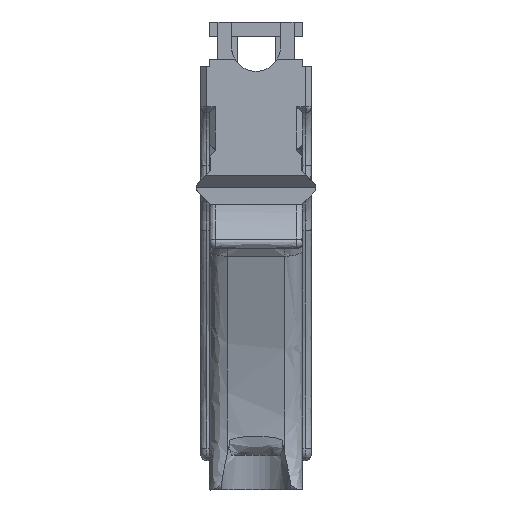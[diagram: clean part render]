
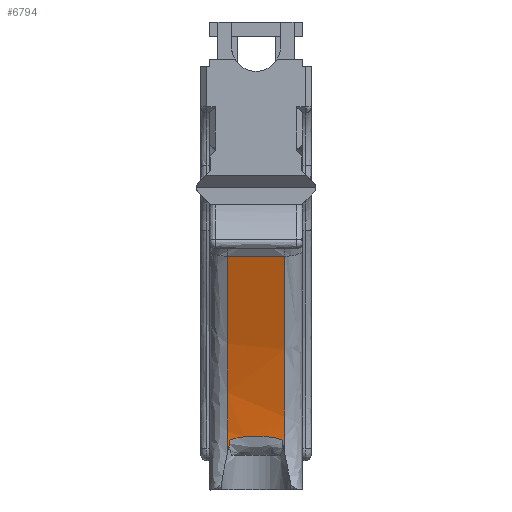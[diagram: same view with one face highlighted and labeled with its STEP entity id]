
A CAD part, front view. The second image highlights one B-rep face of the part: STEP entity #6794.
In plain terms, the highlighted free-form (B-spline) face has degree [5, 1] with [25, 2] control points.
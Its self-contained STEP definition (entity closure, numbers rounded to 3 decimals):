
#52=(
BOUNDED_SURFACE()
B_SPLINE_SURFACE(5,1,((#10452,#10453),(#10454,#10455),(#10456,#10457),(#10458,
#10459),(#10460,#10461),(#10462,#10463),(#10464,#10465),(#10466,#10467),
(#10468,#10469),(#10470,#10471),(#10472,#10473),(#10474,#10475),(#10476,
#10477),(#10478,#10479),(#10480,#10481),(#10482,#10483),(#10484,#10485),
(#10486,#10487),(#10488,#10489),(#10490,#10491),(#10492,#10493),(#10494,
#10495),(#10496,#10497),(#10498,#10499),(#10500,#10501)),.UNSPECIFIED.,
 .F.,.F.,.F.)
B_SPLINE_SURFACE_WITH_KNOTS((6,5,1,1,1,1,1,1,1,1,1,5,6),(2,2),(-1.404,
0.,0.1,0.2,0.3,0.4,0.5,0.6,0.7,0.8,0.9,1.,1.483),(-0.318,
1.908),.UNSPECIFIED.)
GEOMETRIC_REPRESENTATION_ITEM()
RATIONAL_B_SPLINE_SURFACE(((1.,1.),(1.,1.),(1.,1.),(1.,1.),(1.,1.),(1.,
1.),(1.,1.),(1.,1.),(1.,1.),(1.,1.),(1.,1.),(1.,1.),(1.,1.),(1.,1.),(1.,
1.),(1.,1.),(1.,1.),(1.,1.),(1.,1.),(1.,1.),(1.,1.),(1.,1.),(1.,1.),(1.,
1.),(1.,1.)))
REPRESENTATION_ITEM('')
SURFACE()
);
#1772=FACE_OUTER_BOUND('',#2156,.T.);
#2156=EDGE_LOOP('',(#4814,#4815,#4816,#4817,#4818,#4819));
#2686=B_SPLINE_CURVE_WITH_KNOTS('',3,(#9430,#9431,#9432,#9433,#9434,#9435,
#9436,#9437,#9438),.UNSPECIFIED.,.F.,.F.,(4,1,1,1,1,1,4),(-0.959,
-0.877,-0.755,-0.632,-0.386,
-0.141,-0.059),.UNSPECIFIED.);
#2689=B_SPLINE_CURVE_WITH_KNOTS('',3,(#9540,#9541,#9542,#9543,#9544,#9545,
#9546),.UNSPECIFIED.,.F.,.F.,(4,1,1,1,4),(0.582,1.126,
1.749,2.995,4.241),.UNSPECIFIED.);
#2712=B_SPLINE_CURVE_WITH_KNOTS('',3,(#10276,#10277,#10278,#10279,#10280,
#10281,#10282),.UNSPECIFIED.,.F.,.F.,(4,1,1,1,4),(-4.241,-2.995,
-1.749,-1.126,-0.582),.UNSPECIFIED.);
#2723=B_SPLINE_CURVE_WITH_KNOTS('',3,(#10432,#10433,#10434,#10435),
 .UNSPECIFIED.,.F.,.F.,(4,4),(-0.911,-0.711),
 .UNSPECIFIED.);
#2724=B_SPLINE_CURVE_WITH_KNOTS('',3,(#10436,#10437,#10438,#10439),
 .UNSPECIFIED.,.F.,.F.,(4,4),(-0.243,0.),.UNSPECIFIED.);
#2726=B_SPLINE_CURVE_WITH_KNOTS('',3,(#10502,#10503,#10504,#10505),
 .UNSPECIFIED.,.F.,.F.,(4,4),(-1.29,-0.3),
 .UNSPECIFIED.);
#2868=VERTEX_POINT('',#9375);
#2870=VERTEX_POINT('',#9429);
#2872=VERTEX_POINT('',#9533);
#2874=VERTEX_POINT('',#9539);
#3014=VERTEX_POINT('',#10199);
#3019=VERTEX_POINT('',#10274);
#3532=EDGE_CURVE('',#2868,#2870,#2686,.T.);
#3536=EDGE_CURVE('',#2872,#2874,#2689,.T.);
#3699=EDGE_CURVE('',#3019,#3014,#2712,.T.);
#3713=EDGE_CURVE('',#3014,#2868,#2723,.T.);
#3714=EDGE_CURVE('',#2870,#2872,#2724,.T.);
#3717=EDGE_CURVE('',#2874,#3019,#2726,.T.);
#4814=ORIENTED_EDGE('',*,*,#3713,.F.);
#4815=ORIENTED_EDGE('',*,*,#3699,.F.);
#4816=ORIENTED_EDGE('',*,*,#3717,.F.);
#4817=ORIENTED_EDGE('',*,*,#3536,.F.);
#4818=ORIENTED_EDGE('',*,*,#3714,.F.);
#4819=ORIENTED_EDGE('',*,*,#3532,.F.);
#6794=ADVANCED_FACE('',(#1772),#52,.F.);
#9375=CARTESIAN_POINT('',(12.379,-27.933,-61.535));
#9429=CARTESIAN_POINT('',(3.521,-27.933,-61.535));
#9430=CARTESIAN_POINT('Ctrl Pts',(12.379,-27.933,-61.535));
#9431=CARTESIAN_POINT('Ctrl Pts',(12.129,-27.934,-61.435));
#9432=CARTESIAN_POINT('Ctrl Pts',(11.484,-27.939,-61.226));
#9433=CARTESIAN_POINT('Ctrl Pts',(10.413,-27.946,-61.033));
#9434=CARTESIAN_POINT('Ctrl Pts',(8.771,-27.95,-60.907));
#9435=CARTESIAN_POINT('Ctrl Pts',(6.718,-27.951,-60.907));
#9436=CARTESIAN_POINT('Ctrl Pts',(4.803,-27.942,-61.102));
#9437=CARTESIAN_POINT('Ctrl Pts',(3.77,-27.934,-61.435));
#9438=CARTESIAN_POINT('Ctrl Pts',(3.521,-27.933,-61.535));
#9533=CARTESIAN_POINT('',(3.,-28.025,-64.081));
#9539=CARTESIAN_POINT('',(3.,-36.357,-30.134));
#9540=CARTESIAN_POINT('Ctrl Pts',(3.,-28.025,-64.081));
#9541=CARTESIAN_POINT('Ctrl Pts',(3.,-27.873,-62.524));
#9542=CARTESIAN_POINT('Ctrl Pts',(3.,-27.952,-58.998));
#9543=CARTESIAN_POINT('Ctrl Pts',(3.,-29.234,-51.471));
#9544=CARTESIAN_POINT('Ctrl Pts',(3.,-32.102,-41.689));
#9545=CARTESIAN_POINT('Ctrl Pts',(3.,-34.885,-33.975));
#9546=CARTESIAN_POINT('Ctrl Pts',(3.,-36.357,-30.134));
#10199=CARTESIAN_POINT('',(12.9,-28.025,-64.081));
#10274=CARTESIAN_POINT('',(12.9,-36.357,-30.134));
#10276=CARTESIAN_POINT('Ctrl Pts',(12.9,-36.357,-30.134));
#10277=CARTESIAN_POINT('Ctrl Pts',(12.9,-34.885,-33.976));
#10278=CARTESIAN_POINT('Ctrl Pts',(12.9,-32.101,-41.691));
#10279=CARTESIAN_POINT('Ctrl Pts',(12.9,-29.234,-51.473));
#10280=CARTESIAN_POINT('Ctrl Pts',(12.9,-27.951,-59.002));
#10281=CARTESIAN_POINT('Ctrl Pts',(12.9,-27.874,-62.525));
#10282=CARTESIAN_POINT('Ctrl Pts',(12.9,-28.026,-64.08));
#10432=CARTESIAN_POINT('Ctrl Pts',(12.9,-28.025,-64.081));
#10433=CARTESIAN_POINT('Ctrl Pts',(12.725,-27.948,-63.278));
#10434=CARTESIAN_POINT('Ctrl Pts',(12.546,-27.917,-62.431));
#10435=CARTESIAN_POINT('Ctrl Pts',(12.379,-27.933,-61.535));
#10436=CARTESIAN_POINT('Ctrl Pts',(3.521,-27.933,-61.535));
#10437=CARTESIAN_POINT('Ctrl Pts',(3.351,-27.917,-62.445));
#10438=CARTESIAN_POINT('Ctrl Pts',(3.172,-27.949,-63.291));
#10439=CARTESIAN_POINT('Ctrl Pts',(3.,-28.025,-64.081));
#10452=CARTESIAN_POINT('Ctrl Pts',(-3.18,-48.861,
-96.18));
#10453=CARTESIAN_POINT('Ctrl Pts',(19.08,-48.861,-96.18));
#10454=CARTESIAN_POINT('Ctrl Pts',(-3.18,-45.092,
-90.944));
#10455=CARTESIAN_POINT('Ctrl Pts',(19.08,-45.092,-90.944));
#10456=CARTESIAN_POINT('Ctrl Pts',(-3.18,-41.323,
-85.709));
#10457=CARTESIAN_POINT('Ctrl Pts',(19.08,-41.323,-85.709));
#10458=CARTESIAN_POINT('Ctrl Pts',(-3.18,-37.554,
-80.474));
#10459=CARTESIAN_POINT('Ctrl Pts',(19.08,-37.554,-80.474));
#10460=CARTESIAN_POINT('Ctrl Pts',(-3.18,-33.785,
-75.238));
#10461=CARTESIAN_POINT('Ctrl Pts',(19.08,-33.785,-75.238));
#10462=CARTESIAN_POINT('Ctrl Pts',(-3.18,-30.016,
-70.003));
#10463=CARTESIAN_POINT('Ctrl Pts',(19.08,-30.016,-70.003));
#10464=CARTESIAN_POINT('Ctrl Pts',(-3.18,-29.748,
-69.63));
#10465=CARTESIAN_POINT('Ctrl Pts',(19.08,-29.748,-69.63));
#10466=CARTESIAN_POINT('Ctrl Pts',(-3.18,-29.253,
-68.836));
#10467=CARTESIAN_POINT('Ctrl Pts',(19.08,-29.253,-68.836));
#10468=CARTESIAN_POINT('Ctrl Pts',(-3.18,-28.637,
-67.498));
#10469=CARTESIAN_POINT('Ctrl Pts',(19.08,-28.637,-67.498));
#10470=CARTESIAN_POINT('Ctrl Pts',(-3.18,-28.071,
-65.416));
#10471=CARTESIAN_POINT('Ctrl Pts',(19.08,-28.071,-65.416));
#10472=CARTESIAN_POINT('Ctrl Pts',(-3.18,-27.812,
-62.291));
#10473=CARTESIAN_POINT('Ctrl Pts',(19.08,-27.812,-62.291));
#10474=CARTESIAN_POINT('Ctrl Pts',(-3.18,-28.022,
-58.621));
#10475=CARTESIAN_POINT('Ctrl Pts',(19.08,-28.022,-58.621));
#10476=CARTESIAN_POINT('Ctrl Pts',(-3.18,-28.695,-54.412));
#10477=CARTESIAN_POINT('Ctrl Pts',(19.08,-28.695,-54.412));
#10478=CARTESIAN_POINT('Ctrl Pts',(-3.18,-29.793,
-49.709));
#10479=CARTESIAN_POINT('Ctrl Pts',(19.08,-29.793,-49.709));
#10480=CARTESIAN_POINT('Ctrl Pts',(-3.18,-31.267,
-44.567));
#10481=CARTESIAN_POINT('Ctrl Pts',(19.08,-31.267,-44.567));
#10482=CARTESIAN_POINT('Ctrl Pts',(-3.18,-33.073,
-39.04));
#10483=CARTESIAN_POINT('Ctrl Pts',(19.08,-33.073,-39.04));
#10484=CARTESIAN_POINT('Ctrl Pts',(-3.18,-34.754,
-34.343));
#10485=CARTESIAN_POINT('Ctrl Pts',(19.08,-34.754,-34.343));
#10486=CARTESIAN_POINT('Ctrl Pts',(-3.18,-36.138,
-30.676));
#10487=CARTESIAN_POINT('Ctrl Pts',(19.08,-36.138,-30.676));
#10488=CARTESIAN_POINT('Ctrl Pts',(-3.18,-37.114,
-28.169));
#10489=CARTESIAN_POINT('Ctrl Pts',(19.08,-37.114,-28.169));
#10490=CARTESIAN_POINT('Ctrl Pts',(-3.18,-37.616,
-26.9));
#10491=CARTESIAN_POINT('Ctrl Pts',(19.08,-37.616,-26.9));
#10492=CARTESIAN_POINT('Ctrl Pts',(-3.18,-40.039,
-20.77));
#10493=CARTESIAN_POINT('Ctrl Pts',(19.08,-40.039,-20.77));
#10494=CARTESIAN_POINT('Ctrl Pts',(-3.18,-42.463,
-14.639));
#10495=CARTESIAN_POINT('Ctrl Pts',(19.08,-42.463,-14.639));
#10496=CARTESIAN_POINT('Ctrl Pts',(-3.18,-44.886,
-8.508));
#10497=CARTESIAN_POINT('Ctrl Pts',(19.08,-44.886,-8.508));
#10498=CARTESIAN_POINT('Ctrl Pts',(-3.18,-47.31,
-2.377));
#10499=CARTESIAN_POINT('Ctrl Pts',(19.08,-47.31,-2.377));
#10500=CARTESIAN_POINT('Ctrl Pts',(-3.18,-49.733,
3.753));
#10501=CARTESIAN_POINT('Ctrl Pts',(19.08,-49.733,3.753));
#10502=CARTESIAN_POINT('Ctrl Pts',(3.,-36.357,-30.134));
#10503=CARTESIAN_POINT('Ctrl Pts',(6.3,-36.357,-30.134));
#10504=CARTESIAN_POINT('Ctrl Pts',(9.6,-36.357,-30.134));
#10505=CARTESIAN_POINT('Ctrl Pts',(12.9,-36.357,-30.134));
